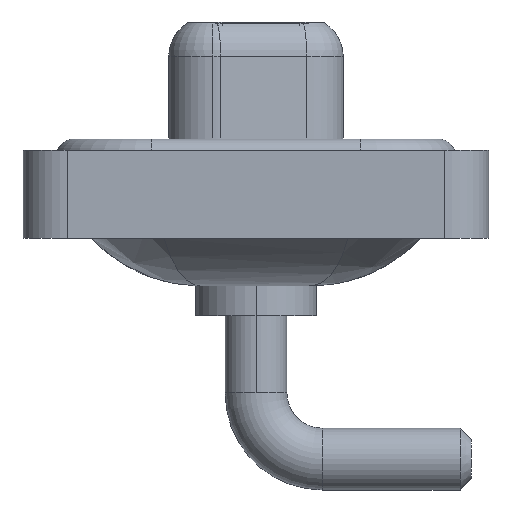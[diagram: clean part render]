
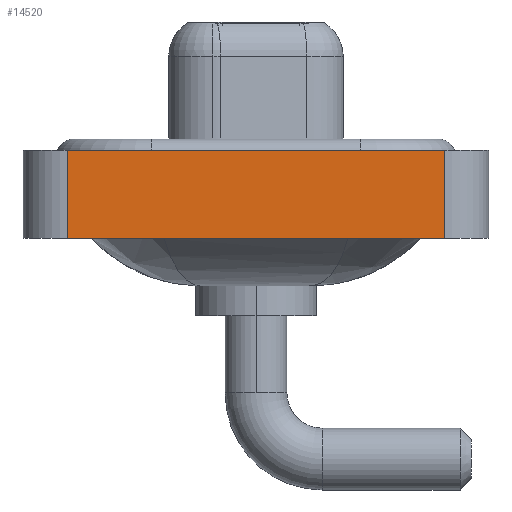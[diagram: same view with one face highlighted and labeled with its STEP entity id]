
A CAD part, left-side view. The second image highlights one B-rep face of the part: STEP entity #14520.
In plain terms, the highlighted planar face has unit normal (-1, 0, 0).
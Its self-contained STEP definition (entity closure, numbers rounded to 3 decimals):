
#986 = VECTOR ( 'NONE', #1534, 1000. ) ;
#1534 = DIRECTION ( 'NONE',  ( 0., 0., 1. ) ) ;
#1631 = VERTEX_POINT ( 'NONE', #5131 ) ;
#2229 = VECTOR ( 'NONE', #13422, 1000. ) ;
#2379 = CARTESIAN_POINT ( 'NONE',  ( -7.25, -8.55, 0.4 ) ) ;
#2450 = EDGE_CURVE ( 'NONE', #13085, #1631, #8568, .T. ) ;
#2746 = CARTESIAN_POINT ( 'NONE',  ( -7.25, 8.55, 0.4 ) ) ;
#3379 = VERTEX_POINT ( 'NONE', #2746 ) ;
#3672 = VECTOR ( 'NONE', #6023, 1000. ) ;
#3825 = VERTEX_POINT ( 'NONE', #10894 ) ;
#4046 = FACE_OUTER_BOUND ( 'NONE', #8922, .T. ) ;
#5131 = CARTESIAN_POINT ( 'NONE',  ( -7.25, -8.55, -3.6 ) ) ;
#5603 = EDGE_CURVE ( 'NONE', #13085, #3379, #13707, .T. ) ;
#6023 = DIRECTION ( 'NONE',  ( 0., -1., 0. ) ) ;
#6254 = PLANE ( 'NONE',  #13677 ) ;
#7467 = ORIENTED_EDGE ( 'NONE', *, *, #11369, .F. ) ;
#7663 = DIRECTION ( 'NONE',  ( 0., 0., 1. ) ) ;
#7687 = DIRECTION ( 'NONE',  ( -1., 0., 0. ) ) ;
#7807 = LINE ( 'NONE', #12335, #986 ) ;
#8466 = VECTOR ( 'NONE', #7663, 1000. ) ;
#8568 = LINE ( 'NONE', #14675, #2229 ) ;
#8922 = EDGE_LOOP ( 'NONE', ( #9231, #7467, #13836, #11365 ) ) ;
#8937 = CARTESIAN_POINT ( 'NONE',  ( -7.25, 8.55, -3.6 ) ) ;
#9231 = ORIENTED_EDGE ( 'NONE', *, *, #12148, .T. ) ;
#10894 = CARTESIAN_POINT ( 'NONE',  ( -7.25, -8.55, 0.4 ) ) ;
#11365 = ORIENTED_EDGE ( 'NONE', *, *, #2450, .T. ) ;
#11369 = EDGE_CURVE ( 'NONE', #3379, #3825, #14360, .T. ) ;
#12148 = EDGE_CURVE ( 'NONE', #1631, #3825, #7807, .T. ) ;
#12335 = CARTESIAN_POINT ( 'NONE',  ( -7.25, -8.55, -3.6 ) ) ;
#12553 = DIRECTION ( 'NONE',  ( 0., 0., 1. ) ) ;
#13085 = VERTEX_POINT ( 'NONE', #14121 ) ;
#13422 = DIRECTION ( 'NONE',  ( 0., -1., 0. ) ) ;
#13677 = AXIS2_PLACEMENT_3D ( 'NONE', #13728, #7687, #12553 ) ;
#13707 = LINE ( 'NONE', #8937, #8466 ) ;
#13728 = CARTESIAN_POINT ( 'NONE',  ( -7.25, -8.55, -3.6 ) ) ;
#13836 = ORIENTED_EDGE ( 'NONE', *, *, #5603, .F. ) ;
#14121 = CARTESIAN_POINT ( 'NONE',  ( -7.25, 8.55, -3.6 ) ) ;
#14360 = LINE ( 'NONE', #2379, #3672 ) ;
#14520 = ADVANCED_FACE ( 'NONE', ( #4046 ), #6254, .T. ) ;
#14675 = CARTESIAN_POINT ( 'NONE',  ( -7.25, -8.55, -3.6 ) ) ;
